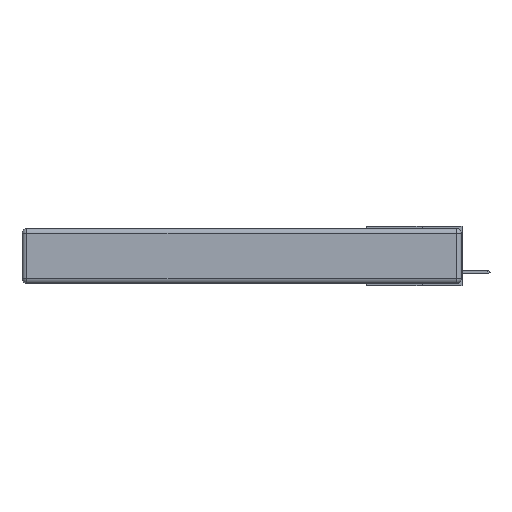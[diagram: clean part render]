
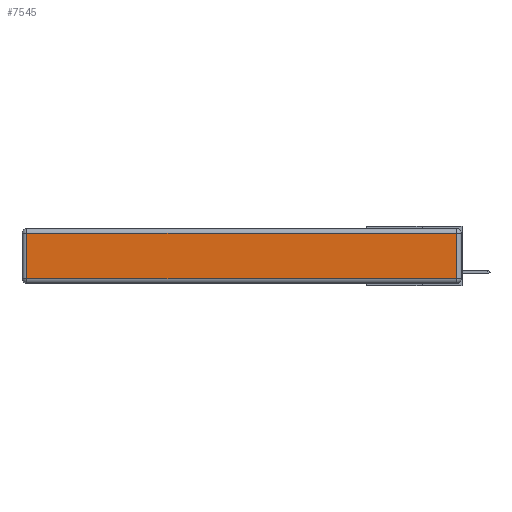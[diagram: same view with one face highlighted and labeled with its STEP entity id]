
A CAD part, left-side view. The second image highlights one B-rep face of the part: STEP entity #7545.
In plain terms, the highlighted planar face has unit normal (-1, 0, 0).
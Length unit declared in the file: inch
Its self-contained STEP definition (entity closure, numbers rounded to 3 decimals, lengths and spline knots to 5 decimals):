
#45 = VECTOR ( 'NONE', #7159, 39.37008 ) ;
#110 = EDGE_CURVE ( 'NONE', #5690, #3018, #316, .T. ) ;
#316 = LINE ( 'NONE', #4490, #10371 ) ;
#331 = VECTOR ( 'NONE', #9514, 39.37008 ) ;
#374 = VECTOR ( 'NONE', #12522, 39.37008 ) ;
#977 = CARTESIAN_POINT ( 'NONE',  ( 0., 2.72, -0.343 ) ) ;
#2463 = LINE ( 'NONE', #8528, #331 ) ;
#2659 = AXIS2_PLACEMENT_3D ( 'NONE', #4574, #11368, #4614 ) ;
#3018 = VERTEX_POINT ( 'NONE', #7431 ) ;
#3949 = EDGE_CURVE ( 'NONE', #5201, #8615, #11492, .T. ) ;
#4165 = CARTESIAN_POINT ( 'NONE',  ( 0., 2.72, -0.03 ) ) ;
#4490 = CARTESIAN_POINT ( 'NONE',  ( 0., 0.03, -0.343 ) ) ;
#4567 = CARTESIAN_POINT ( 'NONE',  ( 0., 0.03, -0.313 ) ) ;
#4574 = CARTESIAN_POINT ( 'NONE',  ( 0., 0., -0.343 ) ) ;
#4614 = DIRECTION ( 'NONE',  ( 0., 0., 1. ) ) ;
#4930 = EDGE_CURVE ( 'NONE', #8615, #5690, #5848, .T. ) ;
#5168 = DIRECTION ( 'NONE',  ( 0., 0., 1. ) ) ;
#5201 = VERTEX_POINT ( 'NONE', #4165 ) ;
#5271 = CARTESIAN_POINT ( 'NONE',  ( 0., 0., -0.313 ) ) ;
#5516 = ORIENTED_EDGE ( 'NONE', *, *, #110, .T. ) ;
#5690 = VERTEX_POINT ( 'NONE', #4567 ) ;
#5702 = ORIENTED_EDGE ( 'NONE', *, *, #3949, .T. ) ;
#5848 = LINE ( 'NONE', #5271, #45 ) ;
#7046 = CARTESIAN_POINT ( 'NONE',  ( 0., 2.72, -0.313 ) ) ;
#7159 = DIRECTION ( 'NONE',  ( 0., -1., 0. ) ) ;
#7431 = CARTESIAN_POINT ( 'NONE',  ( 0., 0.03, -0.03 ) ) ;
#7545 = ADVANCED_FACE ( 'NONE', ( #11354 ), #9411, .T. ) ;
#7614 = ORIENTED_EDGE ( 'NONE', *, *, #9260, .T. ) ;
#8528 = CARTESIAN_POINT ( 'NONE',  ( 0., 2.75, -0.03 ) ) ;
#8615 = VERTEX_POINT ( 'NONE', #7046 ) ;
#8888 = EDGE_LOOP ( 'NONE', ( #11378, #5516, #7614, #5702 ) ) ;
#9260 = EDGE_CURVE ( 'NONE', #3018, #5201, #2463, .T. ) ;
#9411 = PLANE ( 'NONE',  #2659 ) ;
#9514 = DIRECTION ( 'NONE',  ( 0., 1., 0. ) ) ;
#10371 = VECTOR ( 'NONE', #5168, 39.37008 ) ;
#11354 = FACE_OUTER_BOUND ( 'NONE', #8888, .T. ) ;
#11368 = DIRECTION ( 'NONE',  ( -1., 0., 0. ) ) ;
#11378 = ORIENTED_EDGE ( 'NONE', *, *, #4930, .T. ) ;
#11492 = LINE ( 'NONE', #977, #374 ) ;
#12522 = DIRECTION ( 'NONE',  ( 0., 0., -1. ) ) ;
